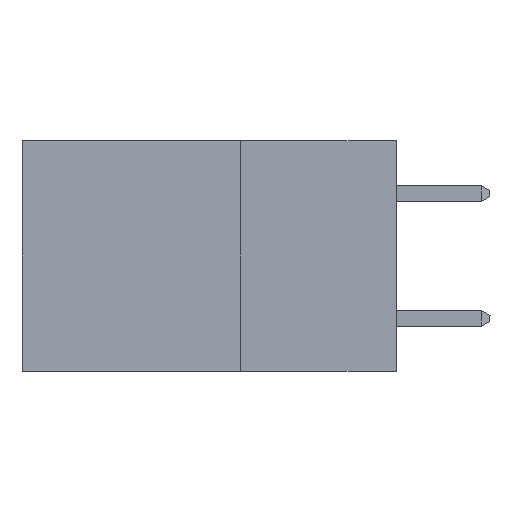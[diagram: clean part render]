
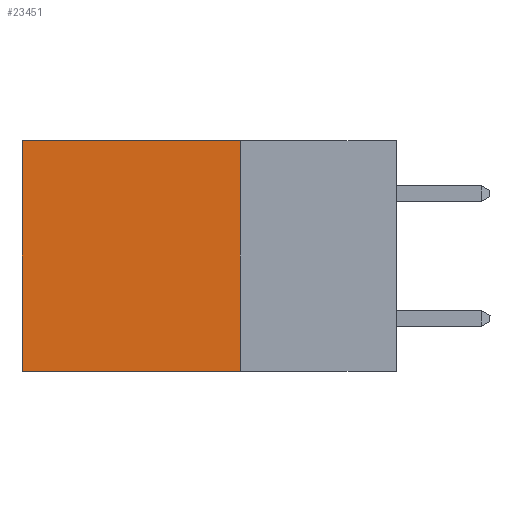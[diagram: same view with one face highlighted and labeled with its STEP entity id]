
A CAD part, left-side view. The second image highlights one B-rep face of the part: STEP entity #23451.
In plain terms, the highlighted planar face has unit normal (-1, 0, 0).
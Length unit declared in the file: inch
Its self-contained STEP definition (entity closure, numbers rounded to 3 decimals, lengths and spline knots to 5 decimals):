
#329 = DIRECTION ( 'NONE',  ( 0., 1., 0. ) ) ;
#1208 = VERTEX_POINT ( 'NONE', #6792 ) ;
#2586 = ORIENTED_EDGE ( 'NONE', *, *, #15066, .F. ) ;
#2609 = ORIENTED_EDGE ( 'NONE', *, *, #9411, .T. ) ;
#3112 = LINE ( 'NONE', #8394, #22553 ) ;
#3234 = CARTESIAN_POINT ( 'NONE',  ( 0.298, 0.6, -0.37 ) ) ;
#3378 = CARTESIAN_POINT ( 'NONE',  ( 0.298, 0.6, 0. ) ) ;
#3920 = ORIENTED_EDGE ( 'NONE', *, *, #17924, .T. ) ;
#4338 = FACE_OUTER_BOUND ( 'NONE', #22307, .T. ) ;
#4607 = EDGE_CURVE ( 'NONE', #12312, #1208, #13571, .T. ) ;
#6792 = CARTESIAN_POINT ( 'NONE',  ( 0.298, 0.25, -0.37 ) ) ;
#7663 = CARTESIAN_POINT ( 'NONE',  ( 0.298, 0.25, 0. ) ) ;
#8394 = CARTESIAN_POINT ( 'NONE',  ( 0.298, 0.25, 0. ) ) ;
#9411 = EDGE_CURVE ( 'NONE', #12312, #23959, #3112, .T. ) ;
#10130 = LINE ( 'NONE', #16044, #12468 ) ;
#11355 = CARTESIAN_POINT ( 'NONE',  ( 0.298, 0.25, 0. ) ) ;
#11370 = DIRECTION ( 'NONE',  ( 0., 0., -1. ) ) ;
#11756 = VERTEX_POINT ( 'NONE', #3234 ) ;
#12040 = DIRECTION ( 'NONE',  ( 0., 1., 0. ) ) ;
#12137 = LINE ( 'NONE', #15126, #18851 ) ;
#12312 = VERTEX_POINT ( 'NONE', #11355 ) ;
#12468 = VECTOR ( 'NONE', #21646, 39.37008 ) ;
#12995 = AXIS2_PLACEMENT_3D ( 'NONE', #7663, #24048, #11370 ) ;
#13156 = VECTOR ( 'NONE', #14548, 39.37008 ) ;
#13571 = LINE ( 'NONE', #14467, #13156 ) ;
#14467 = CARTESIAN_POINT ( 'NONE',  ( 0.298, 0.25, 0. ) ) ;
#14548 = DIRECTION ( 'NONE',  ( 0., 0., -1. ) ) ;
#15066 = EDGE_CURVE ( 'NONE', #1208, #11756, #12137, .T. ) ;
#15126 = CARTESIAN_POINT ( 'NONE',  ( 0.298, 0.25, -0.37 ) ) ;
#16044 = CARTESIAN_POINT ( 'NONE',  ( 0.298, 0.6, 0. ) ) ;
#17223 = ORIENTED_EDGE ( 'NONE', *, *, #4607, .F. ) ;
#17924 = EDGE_CURVE ( 'NONE', #23959, #11756, #10130, .T. ) ;
#18541 = PLANE ( 'NONE',  #12995 ) ;
#18851 = VECTOR ( 'NONE', #329, 39.37008 ) ;
#21646 = DIRECTION ( 'NONE',  ( 0., 0., -1. ) ) ;
#22307 = EDGE_LOOP ( 'NONE', ( #3920, #2586, #17223, #2609 ) ) ;
#22553 = VECTOR ( 'NONE', #12040, 39.37008 ) ;
#23451 = ADVANCED_FACE ( 'NONE', ( #4338 ), #18541, .F. ) ;
#23959 = VERTEX_POINT ( 'NONE', #3378 ) ;
#24048 = DIRECTION ( 'NONE',  ( 1., 0., 0. ) ) ;
